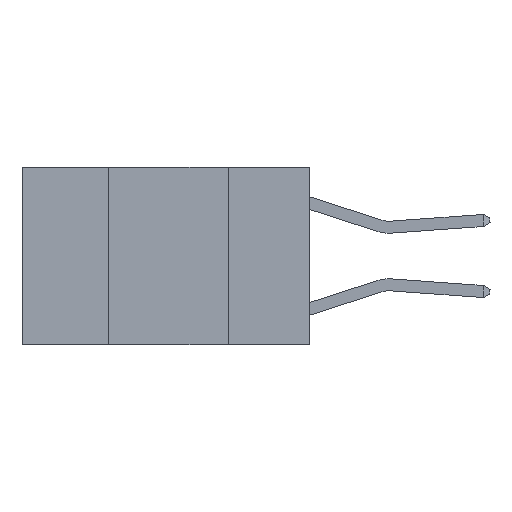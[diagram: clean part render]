
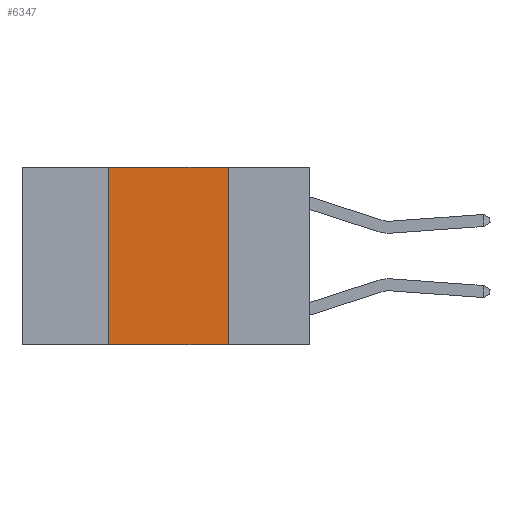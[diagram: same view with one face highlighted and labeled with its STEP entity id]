
A CAD part, left-side view. The second image highlights one B-rep face of the part: STEP entity #6347.
In plain terms, the highlighted planar face has unit normal (-1, 0, 0).
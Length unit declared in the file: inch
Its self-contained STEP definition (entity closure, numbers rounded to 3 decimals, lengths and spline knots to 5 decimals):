
#21 = VERTEX_POINT ( 'NONE', #2023 ) ;
#167 = CARTESIAN_POINT ( 'NONE',  ( 0., 0.42, 0. ) ) ;
#216 = LINE ( 'NONE', #4000, #3885 ) ;
#410 = PLANE ( 'NONE',  #9075 ) ;
#457 = CARTESIAN_POINT ( 'NONE',  ( 0., 0.17, -0.37 ) ) ;
#579 = CARTESIAN_POINT ( 'NONE',  ( 0., 0.6, 0. ) ) ;
#1085 = DIRECTION ( 'NONE',  ( 0., -1., 0. ) ) ;
#2023 = CARTESIAN_POINT ( 'NONE',  ( 0., 0.42, -0.37 ) ) ;
#2374 = EDGE_CURVE ( 'NONE', #21, #7486, #216, .T. ) ;
#2399 = VERTEX_POINT ( 'NONE', #457 ) ;
#2942 = LINE ( 'NONE', #6743, #11400 ) ;
#3885 = VECTOR ( 'NONE', #7778, 39.37008 ) ;
#4000 = CARTESIAN_POINT ( 'NONE',  ( 0., 0.42, 0. ) ) ;
#4194 = CARTESIAN_POINT ( 'NONE',  ( 0., 0.6, 0. ) ) ;
#4369 = DIRECTION ( 'NONE',  ( 0., -1., 0. ) ) ;
#4562 = ORIENTED_EDGE ( 'NONE', *, *, #2374, .F. ) ;
#5157 = LINE ( 'NONE', #579, #12228 ) ;
#5176 = CARTESIAN_POINT ( 'NONE',  ( 0., 0.17, 0. ) ) ;
#5366 = ORIENTED_EDGE ( 'NONE', *, *, #8006, .T. ) ;
#5630 = EDGE_CURVE ( 'NONE', #7486, #6304, #5157, .T. ) ;
#5907 = VECTOR ( 'NONE', #11399, 39.37008 ) ;
#6304 = VERTEX_POINT ( 'NONE', #5176 ) ;
#6347 = ADVANCED_FACE ( 'NONE', ( #10764 ), #410, .F. ) ;
#6405 = ORIENTED_EDGE ( 'NONE', *, *, #5630, .F. ) ;
#6743 = CARTESIAN_POINT ( 'NONE',  ( 0., 0.6, -0.37 ) ) ;
#7308 = EDGE_CURVE ( 'NONE', #6304, #2399, #11213, .T. ) ;
#7486 = VERTEX_POINT ( 'NONE', #167 ) ;
#7619 = CARTESIAN_POINT ( 'NONE',  ( 0., 0.17, 0. ) ) ;
#7778 = DIRECTION ( 'NONE',  ( 0., 0., 1. ) ) ;
#7968 = DIRECTION ( 'NONE',  ( 1., 0., 0. ) ) ;
#8006 = EDGE_CURVE ( 'NONE', #21, #2399, #2942, .T. ) ;
#9075 = AXIS2_PLACEMENT_3D ( 'NONE', #4194, #7968, #9906 ) ;
#9906 = DIRECTION ( 'NONE',  ( 0., 0., -1. ) ) ;
#10474 = ORIENTED_EDGE ( 'NONE', *, *, #7308, .F. ) ;
#10764 = FACE_OUTER_BOUND ( 'NONE', #11217, .T. ) ;
#11213 = LINE ( 'NONE', #7619, #5907 ) ;
#11217 = EDGE_LOOP ( 'NONE', ( #10474, #6405, #4562, #5366 ) ) ;
#11399 = DIRECTION ( 'NONE',  ( 0., 0., -1. ) ) ;
#11400 = VECTOR ( 'NONE', #1085, 39.37008 ) ;
#12228 = VECTOR ( 'NONE', #4369, 39.37008 ) ;
